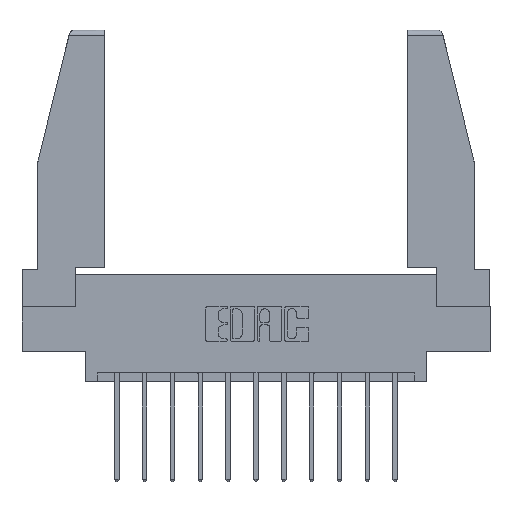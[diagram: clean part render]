
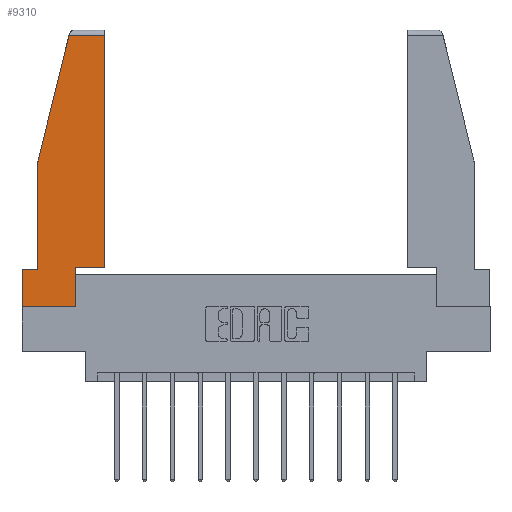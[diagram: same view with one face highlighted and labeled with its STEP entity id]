
A CAD part, top view. The second image highlights one B-rep face of the part: STEP entity #9310.
In plain terms, the highlighted planar face has unit normal (0, 0, 1).
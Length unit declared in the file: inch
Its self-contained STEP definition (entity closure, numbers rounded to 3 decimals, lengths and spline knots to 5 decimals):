
#560 = ORIENTED_EDGE ( 'NONE', *, *, #5560, .T. ) ;
#566 = DIRECTION ( 'NONE',  ( 0., -1., 0. ) ) ;
#878 = VECTOR ( 'NONE', #8118, 39.37008 ) ;
#1058 = LINE ( 'NONE', #1795, #7613 ) ;
#1673 = VECTOR ( 'NONE', #6695, 39.37008 ) ;
#1786 = PLANE ( 'NONE',  #14641 ) ;
#1795 = CARTESIAN_POINT ( 'NONE',  ( 0., 0.21, 0. ) ) ;
#2146 = EDGE_CURVE ( 'NONE', #4272, #8646, #14414, .T. ) ;
#2244 = VERTEX_POINT ( 'NONE', #7053 ) ;
#2302 = CARTESIAN_POINT ( 'NONE',  ( 0.461, 1.52, 0. ) ) ;
#2374 = LINE ( 'NONE', #3422, #14436 ) ;
#2438 = ORIENTED_EDGE ( 'NONE', *, *, #9032, .T. ) ;
#2464 = EDGE_CURVE ( 'NONE', #3175, #6767, #1058, .T. ) ;
#2667 = EDGE_LOOP ( 'NONE', ( #9747, #9728, #14915, #2438, #8698, #4235, #14786, #560, #4627 ) ) ;
#2852 = DIRECTION ( 'NONE',  ( 1., 0., 0. ) ) ;
#3014 = CARTESIAN_POINT ( 'NONE',  ( 0., 0.21, 0. ) ) ;
#3175 = VERTEX_POINT ( 'NONE', #12641 ) ;
#3422 = CARTESIAN_POINT ( 'NONE',  ( 0.297, 0.223, 0. ) ) ;
#3606 = CARTESIAN_POINT ( 'NONE',  ( 0.461, 0.223, 0. ) ) ;
#4235 = ORIENTED_EDGE ( 'NONE', *, *, #4873, .T. ) ;
#4272 = VERTEX_POINT ( 'NONE', #2302 ) ;
#4344 = VERTEX_POINT ( 'NONE', #6155 ) ;
#4488 = CARTESIAN_POINT ( 'NONE',  ( 0.271, 1.55, 0. ) ) ;
#4500 = DIRECTION ( 'NONE',  ( 1., 0., 0. ) ) ;
#4547 = LINE ( 'NONE', #12103, #4906 ) ;
#4627 = ORIENTED_EDGE ( 'NONE', *, *, #5363, .T. ) ;
#4873 = EDGE_CURVE ( 'NONE', #6767, #13808, #5841, .T. ) ;
#4906 = VECTOR ( 'NONE', #8764, 39.37008 ) ;
#5016 = LINE ( 'NONE', #9856, #13970 ) ;
#5363 = EDGE_CURVE ( 'NONE', #2244, #4344, #2374, .T. ) ;
#5480 = CARTESIAN_POINT ( 'NONE',  ( 0., 0.21, 0. ) ) ;
#5560 = EDGE_CURVE ( 'NONE', #11252, #2244, #4547, .T. ) ;
#5841 = LINE ( 'NONE', #5480, #1673 ) ;
#6155 = CARTESIAN_POINT ( 'NONE',  ( 0.461, 0.223, 0. ) ) ;
#6343 = DIRECTION ( 'NONE',  ( 0., 0., 1. ) ) ;
#6529 = VECTOR ( 'NONE', #13530, 39.37008 ) ;
#6684 = LINE ( 'NONE', #3606, #9426 ) ;
#6695 = DIRECTION ( 'NONE',  ( 0., -1., 0. ) ) ;
#6740 = EDGE_CURVE ( 'NONE', #13808, #11252, #8549, .T. ) ;
#6767 = VERTEX_POINT ( 'NONE', #3014 ) ;
#6964 = CARTESIAN_POINT ( 'NONE',  ( 0., 1.52, 0. ) ) ;
#7053 = CARTESIAN_POINT ( 'NONE',  ( 0.297, 0.223, 0. ) ) ;
#7132 = EDGE_CURVE ( 'NONE', #8646, #13989, #7769, .T. ) ;
#7613 = VECTOR ( 'NONE', #10858, 39.37008 ) ;
#7769 = LINE ( 'NONE', #4488, #8899 ) ;
#8078 = CARTESIAN_POINT ( 'NONE',  ( 0.2636, 1.52, 0. ) ) ;
#8118 = DIRECTION ( 'NONE',  ( -1., 0., 0. ) ) ;
#8549 = LINE ( 'NONE', #14822, #6529 ) ;
#8646 = VERTEX_POINT ( 'NONE', #8078 ) ;
#8698 = ORIENTED_EDGE ( 'NONE', *, *, #2464, .T. ) ;
#8764 = DIRECTION ( 'NONE',  ( 0., 1., 0. ) ) ;
#8899 = VECTOR ( 'NONE', #12648, 39.37008 ) ;
#9032 = EDGE_CURVE ( 'NONE', #13989, #3175, #5016, .T. ) ;
#9310 = ADVANCED_FACE ( 'NONE', ( #13425 ), #1786, .T. ) ;
#9426 = VECTOR ( 'NONE', #9532, 39.37008 ) ;
#9532 = DIRECTION ( 'NONE',  ( 0., 1., 0. ) ) ;
#9728 = ORIENTED_EDGE ( 'NONE', *, *, #2146, .T. ) ;
#9747 = ORIENTED_EDGE ( 'NONE', *, *, #10512, .T. ) ;
#9856 = CARTESIAN_POINT ( 'NONE',  ( 0.086, 0.8, 0. ) ) ;
#10512 = EDGE_CURVE ( 'NONE', #4344, #4272, #6684, .T. ) ;
#10858 = DIRECTION ( 'NONE',  ( -1., 0., 0. ) ) ;
#11252 = VERTEX_POINT ( 'NONE', #12932 ) ;
#12103 = CARTESIAN_POINT ( 'NONE',  ( 0.297, 0., 0. ) ) ;
#12140 = CARTESIAN_POINT ( 'NONE',  ( 0., 0., 0. ) ) ;
#12308 = CARTESIAN_POINT ( 'NONE',  ( 0., 0., 0. ) ) ;
#12641 = CARTESIAN_POINT ( 'NONE',  ( 0.086, 0.21, 0. ) ) ;
#12648 = DIRECTION ( 'NONE',  ( -0.239, -0.971, 0. ) ) ;
#12932 = CARTESIAN_POINT ( 'NONE',  ( 0.297, 0., 0. ) ) ;
#13077 = CARTESIAN_POINT ( 'NONE',  ( 0.086, 0.8, 0. ) ) ;
#13425 = FACE_OUTER_BOUND ( 'NONE', #2667, .T. ) ;
#13530 = DIRECTION ( 'NONE',  ( 1., 0., 0. ) ) ;
#13808 = VERTEX_POINT ( 'NONE', #12308 ) ;
#13970 = VECTOR ( 'NONE', #566, 39.37008 ) ;
#13989 = VERTEX_POINT ( 'NONE', #13077 ) ;
#14414 = LINE ( 'NONE', #6964, #878 ) ;
#14436 = VECTOR ( 'NONE', #4500, 39.37008 ) ;
#14641 = AXIS2_PLACEMENT_3D ( 'NONE', #12140, #6343, #2852 ) ;
#14786 = ORIENTED_EDGE ( 'NONE', *, *, #6740, .T. ) ;
#14822 = CARTESIAN_POINT ( 'NONE',  ( 0., 0., 0. ) ) ;
#14915 = ORIENTED_EDGE ( 'NONE', *, *, #7132, .T. ) ;
